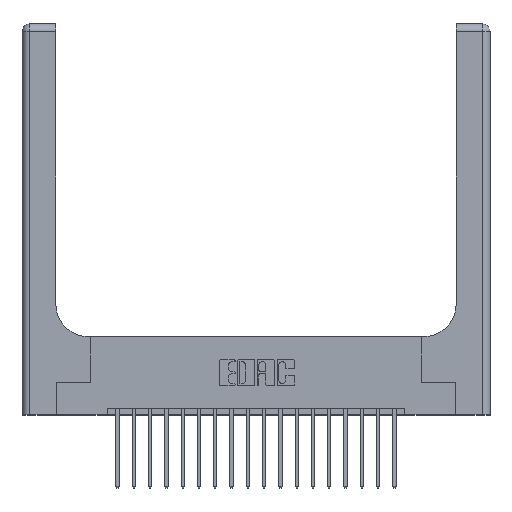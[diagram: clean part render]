
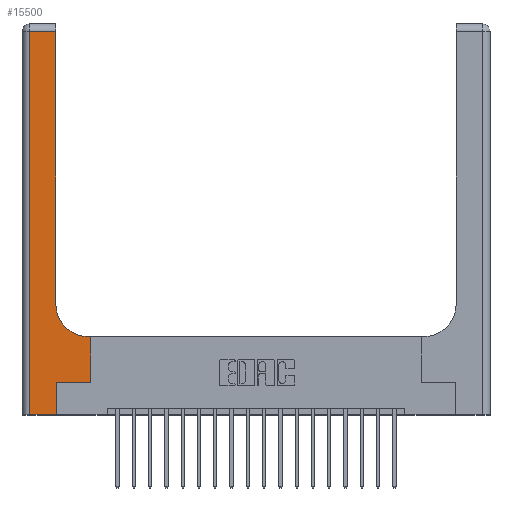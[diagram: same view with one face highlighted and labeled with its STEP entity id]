
A CAD part, top view. The second image highlights one B-rep face of the part: STEP entity #15500.
In plain terms, the highlighted planar face has unit normal (0, 0, 1).
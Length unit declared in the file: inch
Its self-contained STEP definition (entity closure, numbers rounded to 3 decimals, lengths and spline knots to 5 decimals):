
#117 = EDGE_CURVE ( 'NONE', #4401, #19027, #18146, .T. ) ;
#303 = DIRECTION ( 'NONE',  ( 0., 1., 0. ) ) ;
#1189 = CARTESIAN_POINT ( 'NONE',  ( 0.26, 0.6, 0.37 ) ) ;
#1197 = FACE_OUTER_BOUND ( 'NONE', #2177, .T. ) ;
#1741 = EDGE_CURVE ( 'NONE', #15345, #18675, #14129, .T. ) ;
#1784 = VERTEX_POINT ( 'NONE', #19394 ) ;
#1787 = CARTESIAN_POINT ( 'NONE',  ( 0.528, 0.25, 0.37 ) ) ;
#1910 = ORIENTED_EDGE ( 'NONE', *, *, #6909, .T. ) ;
#2177 = EDGE_LOOP ( 'NONE', ( #2313, #13083, #19251, #13635, #6558, #15606, #16894, #1910, #16301 ) ) ;
#2313 = ORIENTED_EDGE ( 'NONE', *, *, #7611, .T. ) ;
#2962 = CARTESIAN_POINT ( 'NONE',  ( 0.528, 0.25, 0.37 ) ) ;
#3305 = EDGE_CURVE ( 'NONE', #19270, #15345, #9500, .T. ) ;
#3336 = CARTESIAN_POINT ( 'NONE',  ( 0.265, 0., 0.37 ) ) ;
#3420 = VECTOR ( 'NONE', #10536, 39.37008 ) ;
#3805 = LINE ( 'NONE', #8194, #15158 ) ;
#3854 = DIRECTION ( 'NONE',  ( -1., 0., 0. ) ) ;
#4176 = CARTESIAN_POINT ( 'NONE',  ( 0.26, 3., 0.37 ) ) ;
#4239 = CARTESIAN_POINT ( 'NONE',  ( 0., 2.94, 0.37 ) ) ;
#4401 = VERTEX_POINT ( 'NONE', #20176 ) ;
#4823 = DIRECTION ( 'NONE',  ( 0., 0., -1. ) ) ;
#5301 = EDGE_CURVE ( 'NONE', #18675, #9943, #7894, .T. ) ;
#6120 = VECTOR ( 'NONE', #9605, 39.37008 ) ;
#6201 = CARTESIAN_POINT ( 'NONE',  ( 0., 3., 0.37 ) ) ;
#6558 = ORIENTED_EDGE ( 'NONE', *, *, #1741, .T. ) ;
#6629 = CARTESIAN_POINT ( 'NONE',  ( 0.06, 0., 0.37 ) ) ;
#6909 = EDGE_CURVE ( 'NONE', #1784, #18810, #20492, .T. ) ;
#7364 = VECTOR ( 'NONE', #7784, 39.37008 ) ;
#7466 = DIRECTION ( 'NONE',  ( 0., 0., -1. ) ) ;
#7611 = EDGE_CURVE ( 'NONE', #15062, #4401, #9179, .T. ) ;
#7784 = DIRECTION ( 'NONE',  ( 1., 0., 0. ) ) ;
#7894 = LINE ( 'NONE', #12409, #7364 ) ;
#8194 = CARTESIAN_POINT ( 'NONE',  ( 0.06, 3., 0.37 ) ) ;
#8668 = CARTESIAN_POINT ( 'NONE',  ( 0.26, 0.85, 0.37 ) ) ;
#8837 = VECTOR ( 'NONE', #13942, 39.37008 ) ;
#9179 = LINE ( 'NONE', #4176, #3420 ) ;
#9500 = LINE ( 'NONE', #15879, #6120 ) ;
#9605 = DIRECTION ( 'NONE',  ( 1., 0., 0. ) ) ;
#9943 = VERTEX_POINT ( 'NONE', #1787 ) ;
#9960 = DIRECTION ( 'NONE',  ( 0., -1., 0. ) ) ;
#10536 = DIRECTION ( 'NONE',  ( 0., 1., 0. ) ) ;
#10882 = DIRECTION ( 'NONE',  ( 0., 1., 0. ) ) ;
#11037 = EDGE_CURVE ( 'NONE', #9943, #1784, #14242, .T. ) ;
#11837 = CIRCLE ( 'NONE', #14837, 0.25 ) ;
#12409 = CARTESIAN_POINT ( 'NONE',  ( 0.265, 0.25, 0.37 ) ) ;
#13083 = ORIENTED_EDGE ( 'NONE', *, *, #117, .T. ) ;
#13254 = CARTESIAN_POINT ( 'NONE',  ( 0.51, 0.6, 0.37 ) ) ;
#13635 = ORIENTED_EDGE ( 'NONE', *, *, #3305, .T. ) ;
#13942 = DIRECTION ( 'NONE',  ( -1., 0., 0. ) ) ;
#14129 = LINE ( 'NONE', #17630, #17672 ) ;
#14242 = LINE ( 'NONE', #2962, #15018 ) ;
#14837 = AXIS2_PLACEMENT_3D ( 'NONE', #19115, #4823, #18069 ) ;
#15018 = VECTOR ( 'NONE', #10882, 39.37008 ) ;
#15062 = VERTEX_POINT ( 'NONE', #8668 ) ;
#15158 = VECTOR ( 'NONE', #9960, 39.37008 ) ;
#15345 = VERTEX_POINT ( 'NONE', #3336 ) ;
#15411 = PLANE ( 'NONE',  #16137 ) ;
#15500 = ADVANCED_FACE ( 'NONE', ( #1197 ), #15411, .F. ) ;
#15514 = DIRECTION ( 'NONE',  ( -1., 0., 0. ) ) ;
#15606 = ORIENTED_EDGE ( 'NONE', *, *, #5301, .T. ) ;
#15879 = CARTESIAN_POINT ( 'NONE',  ( 0., 0., 0.37 ) ) ;
#16137 = AXIS2_PLACEMENT_3D ( 'NONE', #6201, #7466, #15514 ) ;
#16301 = ORIENTED_EDGE ( 'NONE', *, *, #16526, .T. ) ;
#16526 = EDGE_CURVE ( 'NONE', #18810, #15062, #11837, .T. ) ;
#16894 = ORIENTED_EDGE ( 'NONE', *, *, #11037, .T. ) ;
#17616 = CARTESIAN_POINT ( 'NONE',  ( 0.265, 0.25, 0.37 ) ) ;
#17630 = CARTESIAN_POINT ( 'NONE',  ( 0.265, 0., 0.37 ) ) ;
#17672 = VECTOR ( 'NONE', #303, 39.37008 ) ;
#18069 = DIRECTION ( 'NONE',  ( 1., 0., 0. ) ) ;
#18135 = EDGE_CURVE ( 'NONE', #19027, #19270, #3805, .T. ) ;
#18146 = LINE ( 'NONE', #4239, #20250 ) ;
#18541 = CARTESIAN_POINT ( 'NONE',  ( 0.06, 2.94, 0.37 ) ) ;
#18675 = VERTEX_POINT ( 'NONE', #17616 ) ;
#18810 = VERTEX_POINT ( 'NONE', #13254 ) ;
#19027 = VERTEX_POINT ( 'NONE', #18541 ) ;
#19115 = CARTESIAN_POINT ( 'NONE',  ( 0.51, 0.85, 0.37 ) ) ;
#19251 = ORIENTED_EDGE ( 'NONE', *, *, #18135, .T. ) ;
#19270 = VERTEX_POINT ( 'NONE', #6629 ) ;
#19394 = CARTESIAN_POINT ( 'NONE',  ( 0.528, 0.6, 0.37 ) ) ;
#20176 = CARTESIAN_POINT ( 'NONE',  ( 0.26, 2.94, 0.37 ) ) ;
#20250 = VECTOR ( 'NONE', #3854, 39.37008 ) ;
#20492 = LINE ( 'NONE', #1189, #8837 ) ;
